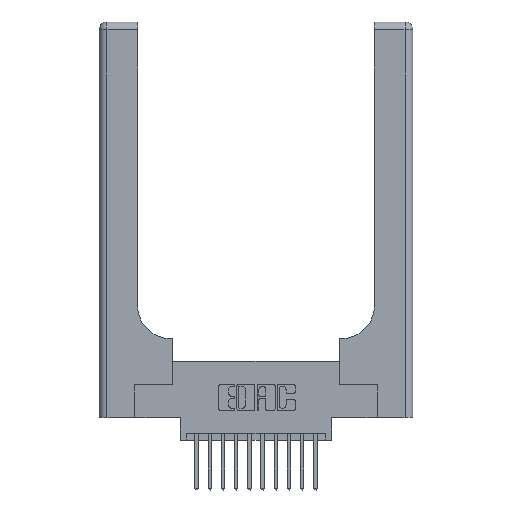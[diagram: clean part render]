
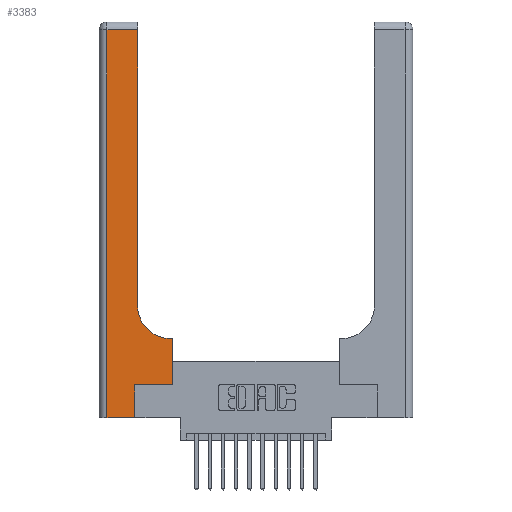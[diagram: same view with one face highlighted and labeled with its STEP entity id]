
A CAD part, top view. The second image highlights one B-rep face of the part: STEP entity #3383.
In plain terms, the highlighted planar face has unit normal (0, 0, 1).
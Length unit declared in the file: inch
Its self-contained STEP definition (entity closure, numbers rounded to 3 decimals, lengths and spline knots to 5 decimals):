
#106 = AXIS2_PLACEMENT_3D ( 'NONE', #13125, #5033, #14446 ) ;
#495 = VERTEX_POINT ( 'NONE', #17424 ) ;
#544 = EDGE_CURVE ( 'NONE', #1914, #15798, #2318, .T. ) ;
#583 = VECTOR ( 'NONE', #15297, 39.37008 ) ;
#732 = CARTESIAN_POINT ( 'NONE',  ( 0.2915, 0.85, 0.37 ) ) ;
#945 = CARTESIAN_POINT ( 'NONE',  ( 0.269, 0.25, 0.37 ) ) ;
#1019 = LINE ( 'NONE', #8610, #583 ) ;
#1084 = VERTEX_POINT ( 'NONE', #3031 ) ;
#1302 = DIRECTION ( 'NONE',  ( -1., 0., 0. ) ) ;
#1427 = EDGE_CURVE ( 'NONE', #15798, #1084, #3170, .T. ) ;
#1529 = EDGE_CURVE ( 'NONE', #1084, #8626, #15771, .T. ) ;
#1850 = VECTOR ( 'NONE', #10139, 39.37008 ) ;
#1914 = VERTEX_POINT ( 'NONE', #732 ) ;
#1934 = CARTESIAN_POINT ( 'NONE',  ( 0., 3., 0.37 ) ) ;
#2318 = LINE ( 'NONE', #17102, #5571 ) ;
#2655 = LINE ( 'NONE', #16409, #8662 ) ;
#2743 = ORIENTED_EDGE ( 'NONE', *, *, #4461, .T. ) ;
#2828 = ORIENTED_EDGE ( 'NONE', *, *, #5796, .T. ) ;
#2857 = VECTOR ( 'NONE', #7029, 39.37008 ) ;
#3031 = CARTESIAN_POINT ( 'NONE',  ( 0.06, 2.94, 0.37 ) ) ;
#3054 = VECTOR ( 'NONE', #3682, 39.37008 ) ;
#3123 = AXIS2_PLACEMENT_3D ( 'NONE', #1934, #11486, #3337 ) ;
#3170 = LINE ( 'NONE', #9298, #10414 ) ;
#3285 = CIRCLE ( 'NONE', #106, 0.25 ) ;
#3337 = DIRECTION ( 'NONE',  ( -1., 0., 0. ) ) ;
#3383 = ADVANCED_FACE ( 'NONE', ( #12684 ), #8785, .F. ) ;
#3433 = ORIENTED_EDGE ( 'NONE', *, *, #15230, .T. ) ;
#3477 = LINE ( 'NONE', #10478, #3054 ) ;
#3533 = ORIENTED_EDGE ( 'NONE', *, *, #5977, .T. ) ;
#3682 = DIRECTION ( 'NONE',  ( 1., 0., 0. ) ) ;
#3703 = ORIENTED_EDGE ( 'NONE', *, *, #11272, .T. ) ;
#4361 = CARTESIAN_POINT ( 'NONE',  ( 0.2915, 2.94, 0.37 ) ) ;
#4461 = EDGE_CURVE ( 'NONE', #9035, #15695, #2655, .T. ) ;
#4965 = ORIENTED_EDGE ( 'NONE', *, *, #12715, .T. ) ;
#5033 = DIRECTION ( 'NONE',  ( 0., 0., -1. ) ) ;
#5221 = CARTESIAN_POINT ( 'NONE',  ( 0.06, 3., 0.37 ) ) ;
#5391 = LINE ( 'NONE', #9802, #12174 ) ;
#5571 = VECTOR ( 'NONE', #16065, 39.37008 ) ;
#5796 = EDGE_CURVE ( 'NONE', #15695, #5931, #5391, .T. ) ;
#5931 = VERTEX_POINT ( 'NONE', #6336 ) ;
#5977 = EDGE_CURVE ( 'NONE', #12094, #9035, #3477, .T. ) ;
#6189 = ORIENTED_EDGE ( 'NONE', *, *, #1529, .T. ) ;
#6204 = ORIENTED_EDGE ( 'NONE', *, *, #544, .T. ) ;
#6336 = CARTESIAN_POINT ( 'NONE',  ( 0.5415, 0.6, 0.37 ) ) ;
#6364 = ORIENTED_EDGE ( 'NONE', *, *, #1427, .T. ) ;
#7029 = DIRECTION ( 'NONE',  ( 1., 0., 0. ) ) ;
#8063 = EDGE_LOOP ( 'NONE', ( #6204, #6364, #6189, #3703, #3433, #3533, #2743, #2828, #4965 ) ) ;
#8610 = CARTESIAN_POINT ( 'NONE',  ( 0.269, 0., 0.37 ) ) ;
#8626 = VERTEX_POINT ( 'NONE', #11685 ) ;
#8662 = VECTOR ( 'NONE', #15147, 39.37008 ) ;
#8785 = PLANE ( 'NONE',  #3123 ) ;
#9035 = VERTEX_POINT ( 'NONE', #15241 ) ;
#9298 = CARTESIAN_POINT ( 'NONE',  ( 0., 2.94, 0.37 ) ) ;
#9802 = CARTESIAN_POINT ( 'NONE',  ( 0.2915, 0.6, 0.37 ) ) ;
#10126 = LINE ( 'NONE', #13709, #2857 ) ;
#10139 = DIRECTION ( 'NONE',  ( 0., -1., 0. ) ) ;
#10414 = VECTOR ( 'NONE', #1302, 39.37008 ) ;
#10478 = CARTESIAN_POINT ( 'NONE',  ( 0.269, 0.25, 0.37 ) ) ;
#10966 = CARTESIAN_POINT ( 'NONE',  ( 0.5585, 0.6, 0.37 ) ) ;
#11272 = EDGE_CURVE ( 'NONE', #8626, #495, #10126, .T. ) ;
#11486 = DIRECTION ( 'NONE',  ( 0., 0., -1. ) ) ;
#11685 = CARTESIAN_POINT ( 'NONE',  ( 0.06, 0., 0.37 ) ) ;
#12094 = VERTEX_POINT ( 'NONE', #945 ) ;
#12174 = VECTOR ( 'NONE', #15401, 39.37008 ) ;
#12684 = FACE_OUTER_BOUND ( 'NONE', #8063, .T. ) ;
#12715 = EDGE_CURVE ( 'NONE', #5931, #1914, #3285, .T. ) ;
#13125 = CARTESIAN_POINT ( 'NONE',  ( 0.5415, 0.85, 0.37 ) ) ;
#13709 = CARTESIAN_POINT ( 'NONE',  ( 0., 0., 0.37 ) ) ;
#14446 = DIRECTION ( 'NONE',  ( 1., 0., 0. ) ) ;
#15147 = DIRECTION ( 'NONE',  ( 0., 1., 0. ) ) ;
#15230 = EDGE_CURVE ( 'NONE', #495, #12094, #1019, .T. ) ;
#15241 = CARTESIAN_POINT ( 'NONE',  ( 0.5585, 0.25, 0.37 ) ) ;
#15297 = DIRECTION ( 'NONE',  ( 0., 1., 0. ) ) ;
#15401 = DIRECTION ( 'NONE',  ( -1., 0., 0. ) ) ;
#15695 = VERTEX_POINT ( 'NONE', #10966 ) ;
#15771 = LINE ( 'NONE', #5221, #1850 ) ;
#15798 = VERTEX_POINT ( 'NONE', #4361 ) ;
#16065 = DIRECTION ( 'NONE',  ( 0., 1., 0. ) ) ;
#16409 = CARTESIAN_POINT ( 'NONE',  ( 0.5585, 0.25, 0.37 ) ) ;
#17102 = CARTESIAN_POINT ( 'NONE',  ( 0.2915, 3., 0.37 ) ) ;
#17424 = CARTESIAN_POINT ( 'NONE',  ( 0.269, 0., 0.37 ) ) ;
